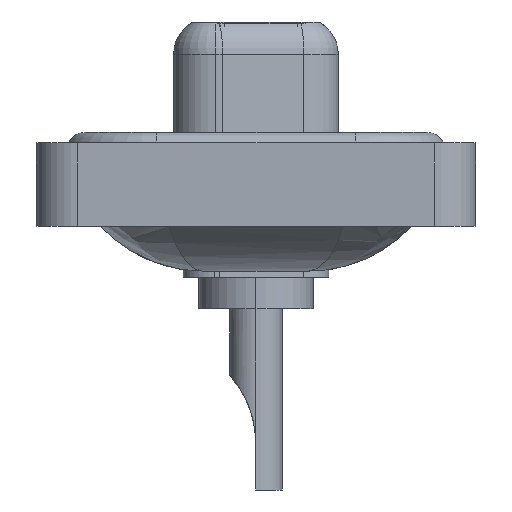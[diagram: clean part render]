
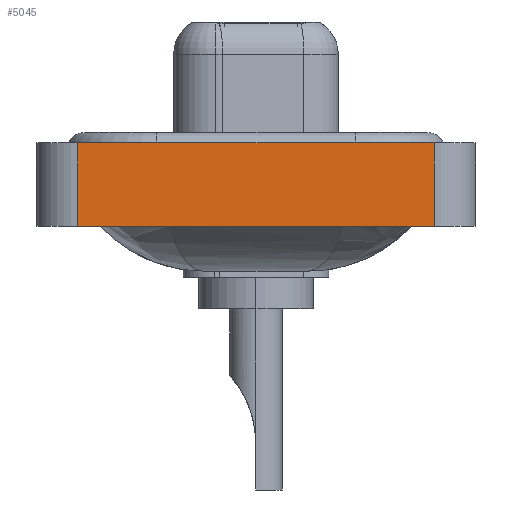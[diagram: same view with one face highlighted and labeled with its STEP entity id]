
A CAD part, left-side view. The second image highlights one B-rep face of the part: STEP entity #5045.
In plain terms, the highlighted planar face has unit normal (-1, 0, 0).
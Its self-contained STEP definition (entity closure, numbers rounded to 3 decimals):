
#117 = CARTESIAN_POINT ( 'NONE',  ( -7.35, 8.55, 0.4 ) ) ;
#223 = VERTEX_POINT ( 'NONE', #117 ) ;
#233 = CARTESIAN_POINT ( 'NONE',  ( -7.35, -8.55, -3.6 ) ) ;
#758 = PLANE ( 'NONE',  #9199 ) ;
#811 = CARTESIAN_POINT ( 'NONE',  ( -7.35, -8.55, 0.4 ) ) ;
#1022 = ORIENTED_EDGE ( 'NONE', *, *, #10234, .F. ) ;
#1086 = VECTOR ( 'NONE', #13365, 1000. ) ;
#1239 = CARTESIAN_POINT ( 'NONE',  ( -7.35, 8.55, -3.6 ) ) ;
#1655 = CARTESIAN_POINT ( 'NONE',  ( -7.35, -8.55, 0.4 ) ) ;
#1926 = VECTOR ( 'NONE', #4735, 1000. ) ;
#2168 = VECTOR ( 'NONE', #8032, 1000. ) ;
#2576 = ORIENTED_EDGE ( 'NONE', *, *, #11780, .F. ) ;
#3266 = DIRECTION ( 'NONE',  ( 0., 0., 1. ) ) ;
#3431 = DIRECTION ( 'NONE',  ( 0., 0., 1. ) ) ;
#3786 = VERTEX_POINT ( 'NONE', #1239 ) ;
#4735 = DIRECTION ( 'NONE',  ( 0., 0., 1. ) ) ;
#5045 = ADVANCED_FACE ( 'NONE', ( #12685 ), #758, .T. ) ;
#5086 = ORIENTED_EDGE ( 'NONE', *, *, #15411, .T. ) ;
#6016 = LINE ( 'NONE', #16390, #1926 ) ;
#6715 = LINE ( 'NONE', #233, #1086 ) ;
#7512 = LINE ( 'NONE', #14922, #13111 ) ;
#7580 = CARTESIAN_POINT ( 'NONE',  ( -7.35, -8.55, -3.6 ) ) ;
#8032 = DIRECTION ( 'NONE',  ( 0., -1., 0. ) ) ;
#8591 = LINE ( 'NONE', #811, #2168 ) ;
#9199 = AXIS2_PLACEMENT_3D ( 'NONE', #7580, #9894, #3431 ) ;
#9894 = DIRECTION ( 'NONE',  ( -1., 0., 0. ) ) ;
#10234 = EDGE_CURVE ( 'NONE', #223, #11245, #8591, .T. ) ;
#11245 = VERTEX_POINT ( 'NONE', #1655 ) ;
#11419 = CARTESIAN_POINT ( 'NONE',  ( -7.35, -8.55, -3.6 ) ) ;
#11780 = EDGE_CURVE ( 'NONE', #3786, #223, #6016, .T. ) ;
#12119 = VERTEX_POINT ( 'NONE', #11419 ) ;
#12236 = EDGE_CURVE ( 'NONE', #12119, #11245, #7512, .T. ) ;
#12277 = ORIENTED_EDGE ( 'NONE', *, *, #12236, .T. ) ;
#12531 = EDGE_LOOP ( 'NONE', ( #12277, #1022, #2576, #5086 ) ) ;
#12685 = FACE_OUTER_BOUND ( 'NONE', #12531, .T. ) ;
#13111 = VECTOR ( 'NONE', #3266, 1000. ) ;
#13365 = DIRECTION ( 'NONE',  ( 0., -1., 0. ) ) ;
#14922 = CARTESIAN_POINT ( 'NONE',  ( -7.35, -8.55, -3.6 ) ) ;
#15411 = EDGE_CURVE ( 'NONE', #3786, #12119, #6715, .T. ) ;
#16390 = CARTESIAN_POINT ( 'NONE',  ( -7.35, 8.55, -3.6 ) ) ;
